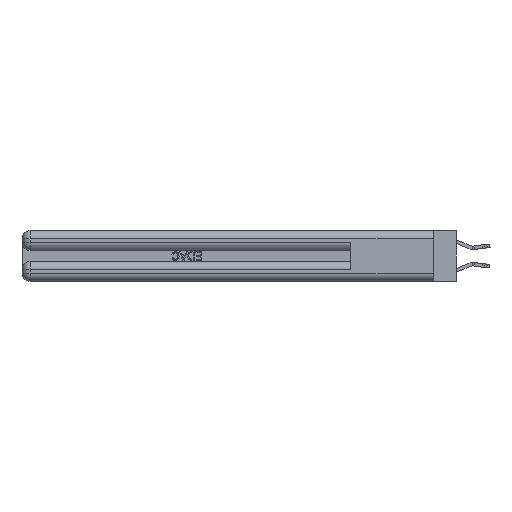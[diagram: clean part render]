
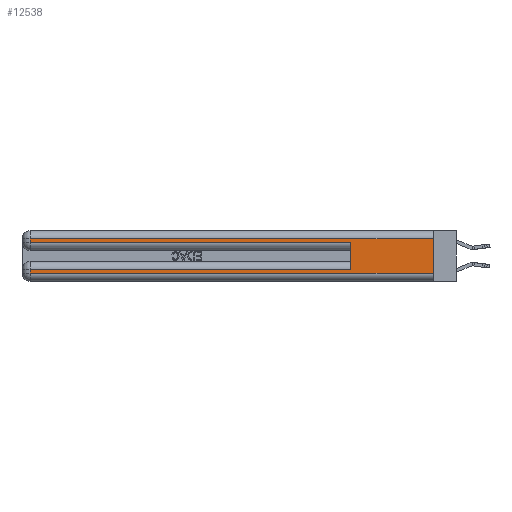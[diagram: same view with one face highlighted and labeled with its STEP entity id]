
A CAD part, left-side view. The second image highlights one B-rep face of the part: STEP entity #12538.
In plain terms, the highlighted planar face has unit normal (-1, 0, 0).
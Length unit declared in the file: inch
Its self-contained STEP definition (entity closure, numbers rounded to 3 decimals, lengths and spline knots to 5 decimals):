
#260 = CARTESIAN_POINT ( 'NONE',  ( 0., 0., 0.31 ) ) ;
#592 = DIRECTION ( 'NONE',  ( 0., 0., 1. ) ) ;
#644 = CARTESIAN_POINT ( 'NONE',  ( 0., 0., 0.06 ) ) ;
#1321 = VERTEX_POINT ( 'NONE', #27685 ) ;
#2165 = ORIENTED_EDGE ( 'NONE', *, *, #8237, .T. ) ;
#2471 = ORIENTED_EDGE ( 'NONE', *, *, #24611, .T. ) ;
#3904 = VERTEX_POINT ( 'NONE', #8458 ) ;
#4216 = LINE ( 'NONE', #7315, #18235 ) ;
#4297 = ORIENTED_EDGE ( 'NONE', *, *, #22711, .T. ) ;
#4859 = CARTESIAN_POINT ( 'NONE',  ( 0., 0., 0.37 ) ) ;
#5421 = CARTESIAN_POINT ( 'NONE',  ( 0., 0., 0.285 ) ) ;
#5705 = CARTESIAN_POINT ( 'NONE',  ( 0., 0., 0.06 ) ) ;
#7315 = CARTESIAN_POINT ( 'NONE',  ( 0., 0., 0.37 ) ) ;
#8181 = VECTOR ( 'NONE', #28148, 39.37008 ) ;
#8237 = EDGE_CURVE ( 'NONE', #8334, #15603, #29488, .T. ) ;
#8334 = VERTEX_POINT ( 'NONE', #29502 ) ;
#8458 = CARTESIAN_POINT ( 'NONE',  ( 0., 0.6, 0.085 ) ) ;
#8993 = LINE ( 'NONE', #17565, #8181 ) ;
#9360 = VERTEX_POINT ( 'NONE', #5705 ) ;
#9673 = LINE ( 'NONE', #33838, #15005 ) ;
#9923 = VERTEX_POINT ( 'NONE', #260 ) ;
#10194 = DIRECTION ( 'NONE',  ( 0., 0., -1. ) ) ;
#10581 = EDGE_CURVE ( 'NONE', #9923, #9360, #4216, .T. ) ;
#11152 = CARTESIAN_POINT ( 'NONE',  ( 0., 2.94, 0.085 ) ) ;
#11353 = VERTEX_POINT ( 'NONE', #21514 ) ;
#12538 = ADVANCED_FACE ( 'NONE', ( #14804 ), #20638, .F. ) ;
#12768 = CARTESIAN_POINT ( 'NONE',  ( 0., 0., 0.31 ) ) ;
#13699 = CARTESIAN_POINT ( 'NONE',  ( 0., 0.6, 0.145 ) ) ;
#14635 = LINE ( 'NONE', #12768, #20805 ) ;
#14804 = FACE_OUTER_BOUND ( 'NONE', #19468, .T. ) ;
#15005 = VECTOR ( 'NONE', #31425, 39.37008 ) ;
#15603 = VERTEX_POINT ( 'NONE', #31998 ) ;
#16100 = ORIENTED_EDGE ( 'NONE', *, *, #23957, .T. ) ;
#16580 = VERTEX_POINT ( 'NONE', #11152 ) ;
#16916 = ORIENTED_EDGE ( 'NONE', *, *, #32079, .F. ) ;
#17153 = EDGE_CURVE ( 'NONE', #11353, #9360, #33239, .T. ) ;
#17565 = CARTESIAN_POINT ( 'NONE',  ( 0., 2.94, 0.37 ) ) ;
#17780 = LINE ( 'NONE', #13699, #23962 ) ;
#18235 = VECTOR ( 'NONE', #25565, 39.37008 ) ;
#19468 = EDGE_LOOP ( 'NONE', ( #26213, #16100, #4297, #2165, #16916, #19573, #2471, #23489 ) ) ;
#19573 = ORIENTED_EDGE ( 'NONE', *, *, #28541, .T. ) ;
#20638 = PLANE ( 'NONE',  #30196 ) ;
#20805 = VECTOR ( 'NONE', #33871, 39.37008 ) ;
#21514 = CARTESIAN_POINT ( 'NONE',  ( 0., 2.94, 0.06 ) ) ;
#22474 = VECTOR ( 'NONE', #26488, 39.37008 ) ;
#22711 = EDGE_CURVE ( 'NONE', #1321, #8334, #8993, .T. ) ;
#22966 = LINE ( 'NONE', #23617, #28301 ) ;
#23489 = ORIENTED_EDGE ( 'NONE', *, *, #17153, .T. ) ;
#23617 = CARTESIAN_POINT ( 'NONE',  ( 0., 0., 0.085 ) ) ;
#23957 = EDGE_CURVE ( 'NONE', #9923, #1321, #14635, .T. ) ;
#23962 = VECTOR ( 'NONE', #592, 39.37008 ) ;
#24337 = DIRECTION ( 'NONE',  ( 0., -1., 0. ) ) ;
#24611 = EDGE_CURVE ( 'NONE', #16580, #11353, #9673, .T. ) ;
#25565 = DIRECTION ( 'NONE',  ( 0., 0., -1. ) ) ;
#25917 = DIRECTION ( 'NONE',  ( 1., 0., 0. ) ) ;
#26208 = VECTOR ( 'NONE', #24337, 39.37008 ) ;
#26213 = ORIENTED_EDGE ( 'NONE', *, *, #10581, .F. ) ;
#26488 = DIRECTION ( 'NONE',  ( 0., -1., 0. ) ) ;
#27685 = CARTESIAN_POINT ( 'NONE',  ( 0., 2.94, 0.31 ) ) ;
#28148 = DIRECTION ( 'NONE',  ( 0., 0., -1. ) ) ;
#28301 = VECTOR ( 'NONE', #29037, 39.37008 ) ;
#28541 = EDGE_CURVE ( 'NONE', #3904, #16580, #22966, .T. ) ;
#29037 = DIRECTION ( 'NONE',  ( 0., 1., 0. ) ) ;
#29488 = LINE ( 'NONE', #5421, #22474 ) ;
#29502 = CARTESIAN_POINT ( 'NONE',  ( 0., 2.94, 0.285 ) ) ;
#30196 = AXIS2_PLACEMENT_3D ( 'NONE', #4859, #25917, #10194 ) ;
#31425 = DIRECTION ( 'NONE',  ( 0., 0., -1. ) ) ;
#31998 = CARTESIAN_POINT ( 'NONE',  ( 0., 0.6, 0.285 ) ) ;
#32079 = EDGE_CURVE ( 'NONE', #3904, #15603, #17780, .T. ) ;
#33239 = LINE ( 'NONE', #644, #26208 ) ;
#33838 = CARTESIAN_POINT ( 'NONE',  ( 0., 2.94, 0.37 ) ) ;
#33871 = DIRECTION ( 'NONE',  ( 0., 1., 0. ) ) ;
